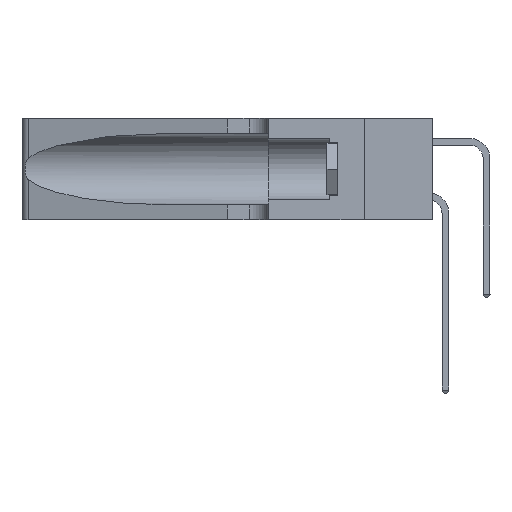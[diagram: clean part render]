
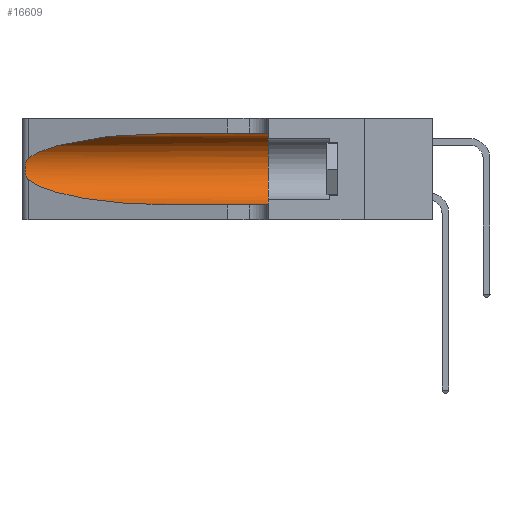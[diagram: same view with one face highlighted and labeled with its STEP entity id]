
A CAD part, left-side view. The second image highlights one B-rep face of the part: STEP entity #16609.
In plain terms, the highlighted cylindrical face has radius 3.308 mm (diameter 6.617 mm), a partial arc.
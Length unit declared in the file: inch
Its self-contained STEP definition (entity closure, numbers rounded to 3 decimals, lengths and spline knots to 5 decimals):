
#478 = CARTESIAN_POINT ( 'NONE',  ( 0.25555, 1.22993, 0.14849 ) ) ;
#1467 = ORIENTED_EDGE ( 'NONE', *, *, #4156, .T. ) ;
#3063 = CARTESIAN_POINT ( 'NONE',  ( 0.25487, 1.22718, 0.22369 ) ) ;
#3260 = VERTEX_POINT ( 'NONE', #3063 ) ;
#3369 = B_SPLINE_CURVE_WITH_KNOTS ( 'NONE', 3,
 ( #20095, #20275, #5663, #13374, #17414, #15858, #15536, #15615, #8433, #10315, #15195, #23389, #478, #15242 ),
 .UNSPECIFIED., .F., .F.,
 ( 4, 2, 2, 2, 2, 2, 4 ),
 ( 0., 0.00027, 0.00053, 0.00107, 0.0016, 0.00187, 0.00214 ),
 .UNSPECIFIED. ) ;
#4123 = CARTESIAN_POINT ( 'NONE',  ( 0.18966, 0.96281, 0.05475 ) ) ;
#4156 = EDGE_CURVE ( 'NONE', #4264, #15264, #16656, .T. ) ;
#4203 = CARTESIAN_POINT ( 'NONE',  ( 0.1305, 0.72297, 0.05475 ) ) ;
#4264 = VERTEX_POINT ( 'NONE', #9957 ) ;
#4302 = CARTESIAN_POINT ( 'NONE',  ( 0.25487, 1.22718, 0.22369 ) ) ;
#4955 = VECTOR ( 'NONE', #19363, 39.37008 ) ;
#5663 = CARTESIAN_POINT ( 'NONE',  ( 0.25639, 1.23184, 0.21858 ) ) ;
#6241 = CARTESIAN_POINT ( 'NONE',  ( 0.2373, 1.15595, 0.08982 ) ) ;
#6467 = CARTESIAN_POINT ( 'NONE',  ( 0.25487, 1.22718, 0.14631 ) ) ;
#7800 = VECTOR ( 'NONE', #20663, 39.37008 ) ;
#8305 = CARTESIAN_POINT ( 'NONE',  ( 0.2373, 1.15595, 0.28018 ) ) ;
#8433 = CARTESIAN_POINT ( 'NONE',  ( 0.26017, 1.23833, 0.17102 ) ) ;
#8593 = EDGE_CURVE ( 'NONE', #22549, #15496, #24041, .T. ) ;
#9015 = ORIENTED_EDGE ( 'NONE', *, *, #13213, .F. ) ;
#9623 = CARTESIAN_POINT ( 'NONE',  ( 0.1305, 0.35, 0.31525 ) ) ;
#9957 = CARTESIAN_POINT ( 'NONE',  ( 0.1305, 0.72297, 0.05475 ) ) ;
#10315 = CARTESIAN_POINT ( 'NONE',  ( 0.25856, 1.23593, 0.16098 ) ) ;
#12042 = ORIENTED_EDGE ( 'NONE', *, *, #15272, .T. ) ;
#12527 = CARTESIAN_POINT ( 'NONE',  ( 0.1305, 1.61858, 0.05475 ) ) ;
#13213 = EDGE_CURVE ( 'NONE', #15496, #15264, #14270, .T. ) ;
#13229 = CYLINDRICAL_SURFACE ( 'NONE', #22927, 0.13025 ) ;
#13374 = CARTESIAN_POINT ( 'NONE',  ( 0.25787, 1.23484, 0.2124 ) ) ;
#14270 = CIRCLE ( 'NONE', #23354, 0.13025 ) ;
#14304 =( BOUNDED_CURVE ( )  B_SPLINE_CURVE ( 3, ( #21515, #6241, #4123, #4203 ),
 .UNSPECIFIED., .F., .F. ) 
 B_SPLINE_CURVE_WITH_KNOTS ( ( 4, 4 ),
 ( 3.44316, 4.71239 ),
 .UNSPECIFIED. ) 
 CURVE ( )  GEOMETRIC_REPRESENTATION_ITEM ( )  RATIONAL_B_SPLINE_CURVE ( ( 1., 0.87, 0.87, 1. ) ) 
 REPRESENTATION_ITEM ( '' )  );
#14311 = CARTESIAN_POINT ( 'NONE',  ( 0.1305, 0.72297, 0.31525 ) ) ;
#14794 = EDGE_LOOP ( 'NONE', ( #17197, #24278, #12042, #1467, #9015, #23996 ) ) ;
#15195 = CARTESIAN_POINT ( 'NONE',  ( 0.25789, 1.23486, 0.15765 ) ) ;
#15242 = CARTESIAN_POINT ( 'NONE',  ( 0.25487, 1.22718, 0.14631 ) ) ;
#15264 = VERTEX_POINT ( 'NONE', #21753 ) ;
#15272 = EDGE_CURVE ( 'NONE', #16693, #4264, #14304, .T. ) ;
#15319 = FACE_OUTER_BOUND ( 'NONE', #14794, .T. ) ;
#15346 = CARTESIAN_POINT ( 'NONE',  ( 0.1305, 1.61858, 0.31525 ) ) ;
#15496 = VERTEX_POINT ( 'NONE', #9623 ) ;
#15536 = CARTESIAN_POINT ( 'NONE',  ( 0.26075, 1.23896, 0.19203 ) ) ;
#15615 = CARTESIAN_POINT ( 'NONE',  ( 0.26075, 1.23896, 0.178 ) ) ;
#15858 = CARTESIAN_POINT ( 'NONE',  ( 0.26018, 1.23835, 0.19895 ) ) ;
#16609 = ADVANCED_FACE ( 'NONE', ( #15319 ), #13229, .F. ) ;
#16656 = LINE ( 'NONE', #12527, #7800 ) ;
#16693 = VERTEX_POINT ( 'NONE', #6467 ) ;
#17161 = DIRECTION ( 'NONE',  ( 0., 1., 0. ) ) ;
#17197 = ORIENTED_EDGE ( 'NONE', *, *, #23256, .T. ) ;
#17414 = CARTESIAN_POINT ( 'NONE',  ( 0.25854, 1.2359, 0.20912 ) ) ;
#17782 = CARTESIAN_POINT ( 'NONE',  ( 0.1305, 0.72297, 0.31525 ) ) ;
#18409 = CARTESIAN_POINT ( 'NONE',  ( 0.1305, 1.61858, 0.185 ) ) ;
#19191 = EDGE_CURVE ( 'NONE', #3260, #16693, #3369, .T. ) ;
#19363 = DIRECTION ( 'NONE',  ( 0., -1., 0. ) ) ;
#20095 = CARTESIAN_POINT ( 'NONE',  ( 0.25487, 1.22718, 0.22369 ) ) ;
#20258 = DIRECTION ( 'NONE',  ( 0., -1., 0. ) ) ;
#20275 = CARTESIAN_POINT ( 'NONE',  ( 0.25555, 1.22994, 0.2215 ) ) ;
#20311 =( BOUNDED_CURVE ( )  B_SPLINE_CURVE ( 3, ( #14311, #22023, #8305, #4302 ),
 .UNSPECIFIED., .F., .F. ) 
 B_SPLINE_CURVE_WITH_KNOTS ( ( 4, 4 ),
 ( 1.5708, 2.84003 ),
 .UNSPECIFIED. ) 
 CURVE ( )  GEOMETRIC_REPRESENTATION_ITEM ( )  RATIONAL_B_SPLINE_CURVE ( ( 1., 0.87, 0.87, 1. ) ) 
 REPRESENTATION_ITEM ( '' )  );
#20663 = DIRECTION ( 'NONE',  ( 0., -1., 0. ) ) ;
#20945 = CARTESIAN_POINT ( 'NONE',  ( 0.1305, 0.35, 0.185 ) ) ;
#21515 = CARTESIAN_POINT ( 'NONE',  ( 0.25487, 1.22718, 0.14631 ) ) ;
#21753 = CARTESIAN_POINT ( 'NONE',  ( 0.1305, 0.35, 0.05475 ) ) ;
#22023 = CARTESIAN_POINT ( 'NONE',  ( 0.18966, 0.96281, 0.31525 ) ) ;
#22549 = VERTEX_POINT ( 'NONE', #17782 ) ;
#22927 = AXIS2_PLACEMENT_3D ( 'NONE', #18409, #20258, #24197 ) ;
#23256 = EDGE_CURVE ( 'NONE', #22549, #3260, #20311, .T. ) ;
#23354 = AXIS2_PLACEMENT_3D ( 'NONE', #20945, #17161, #24808 ) ;
#23389 = CARTESIAN_POINT ( 'NONE',  ( 0.25639, 1.23186, 0.15144 ) ) ;
#23996 = ORIENTED_EDGE ( 'NONE', *, *, #8593, .F. ) ;
#24041 = LINE ( 'NONE', #15346, #4955 ) ;
#24197 = DIRECTION ( 'NONE',  ( 0., 0., -1. ) ) ;
#24278 = ORIENTED_EDGE ( 'NONE', *, *, #19191, .T. ) ;
#24808 = DIRECTION ( 'NONE',  ( 0., 0., 1. ) ) ;
